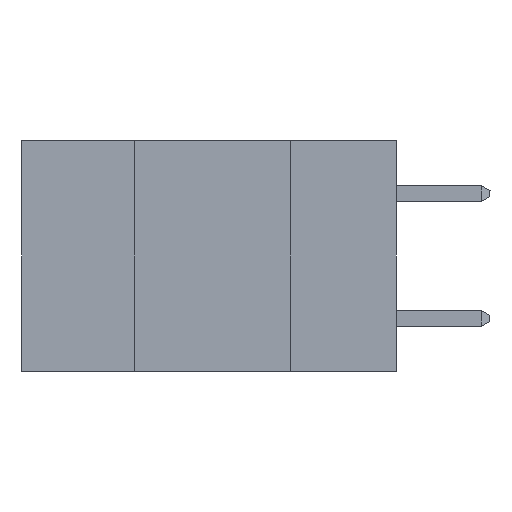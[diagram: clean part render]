
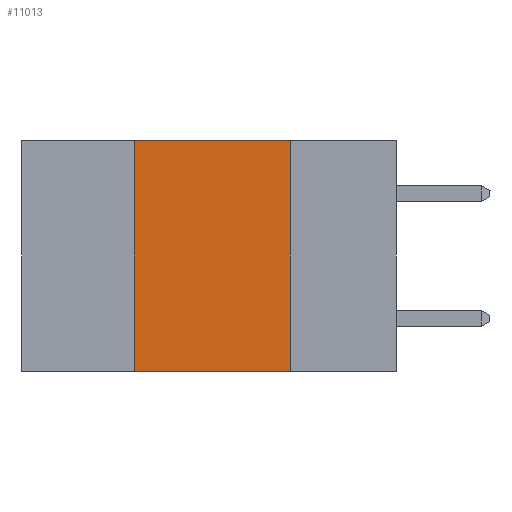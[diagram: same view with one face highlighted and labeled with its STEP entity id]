
A CAD part, left-side view. The second image highlights one B-rep face of the part: STEP entity #11013.
In plain terms, the highlighted planar face has unit normal (-1, 0, 0).
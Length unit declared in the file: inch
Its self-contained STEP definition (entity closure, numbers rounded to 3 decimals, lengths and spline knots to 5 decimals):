
#1648 = ORIENTED_EDGE ( 'NONE', *, *, #12779, .F. ) ;
#3150 = CARTESIAN_POINT ( 'NONE',  ( 0., 0.42, 0. ) ) ;
#4323 = VECTOR ( 'NONE', #24695, 39.37008 ) ;
#5111 = ORIENTED_EDGE ( 'NONE', *, *, #29473, .T. ) ;
#5336 = VERTEX_POINT ( 'NONE', #27675 ) ;
#9018 = ORIENTED_EDGE ( 'NONE', *, *, #17388, .F. ) ;
#9480 = CARTESIAN_POINT ( 'NONE',  ( 0., 0.17, 0. ) ) ;
#11013 = ADVANCED_FACE ( 'NONE', ( #12055 ), #29661, .F. ) ;
#12055 = FACE_OUTER_BOUND ( 'NONE', #13862, .T. ) ;
#12190 = LINE ( 'NONE', #25559, #17780 ) ;
#12604 = EDGE_CURVE ( 'NONE', #26500, #20717, #17170, .T. ) ;
#12779 = EDGE_CURVE ( 'NONE', #20717, #17429, #29917, .T. ) ;
#13503 = VECTOR ( 'NONE', #21260, 39.37008 ) ;
#13862 = EDGE_LOOP ( 'NONE', ( #9018, #1648, #20357, #5111 ) ) ;
#14256 = LINE ( 'NONE', #30453, #13503 ) ;
#15993 = DIRECTION ( 'NONE',  ( 0., -1., 0. ) ) ;
#17170 = LINE ( 'NONE', #3150, #4323 ) ;
#17388 = EDGE_CURVE ( 'NONE', #17429, #5336, #14256, .T. ) ;
#17429 = VERTEX_POINT ( 'NONE', #9480 ) ;
#17780 = VECTOR ( 'NONE', #27886, 39.37008 ) ;
#20357 = ORIENTED_EDGE ( 'NONE', *, *, #12604, .F. ) ;
#20634 = CARTESIAN_POINT ( 'NONE',  ( 0., 0.6, 0. ) ) ;
#20717 = VERTEX_POINT ( 'NONE', #28951 ) ;
#21260 = DIRECTION ( 'NONE',  ( 0., 0., -1. ) ) ;
#23751 = VECTOR ( 'NONE', #15993, 39.37008 ) ;
#23876 = CARTESIAN_POINT ( 'NONE',  ( 0., 0.42, -0.37 ) ) ;
#23901 = CARTESIAN_POINT ( 'NONE',  ( 0., 0.6, 0. ) ) ;
#24695 = DIRECTION ( 'NONE',  ( 0., 0., 1. ) ) ;
#25143 = AXIS2_PLACEMENT_3D ( 'NONE', #23901, #25492, #25389 ) ;
#25389 = DIRECTION ( 'NONE',  ( 0., 0., -1. ) ) ;
#25492 = DIRECTION ( 'NONE',  ( 1., 0., 0. ) ) ;
#25559 = CARTESIAN_POINT ( 'NONE',  ( 0., 0.6, -0.37 ) ) ;
#26500 = VERTEX_POINT ( 'NONE', #23876 ) ;
#27675 = CARTESIAN_POINT ( 'NONE',  ( 0., 0.17, -0.37 ) ) ;
#27886 = DIRECTION ( 'NONE',  ( 0., -1., 0. ) ) ;
#28951 = CARTESIAN_POINT ( 'NONE',  ( 0., 0.42, 0. ) ) ;
#29473 = EDGE_CURVE ( 'NONE', #26500, #5336, #12190, .T. ) ;
#29661 = PLANE ( 'NONE',  #25143 ) ;
#29917 = LINE ( 'NONE', #20634, #23751 ) ;
#30453 = CARTESIAN_POINT ( 'NONE',  ( 0., 0.17, 0. ) ) ;
